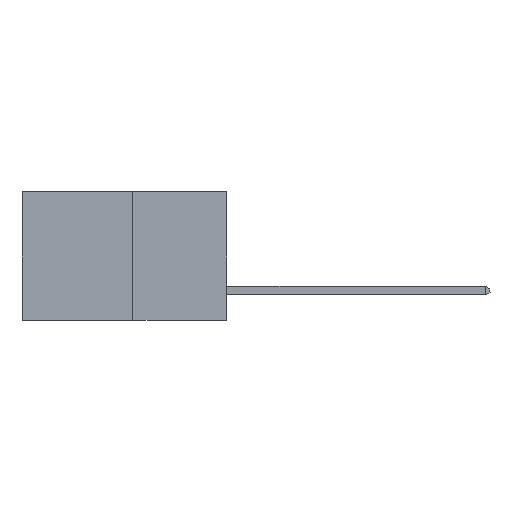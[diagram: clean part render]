
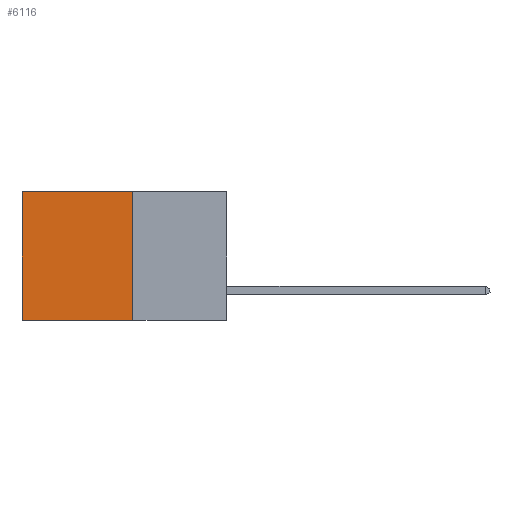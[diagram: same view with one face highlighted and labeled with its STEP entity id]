
A CAD part, left-side view. The second image highlights one B-rep face of the part: STEP entity #6116.
In plain terms, the highlighted planar face has unit normal (-1, 0, 0).
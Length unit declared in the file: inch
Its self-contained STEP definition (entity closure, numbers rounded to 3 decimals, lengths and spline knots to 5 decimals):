
#478 = LINE ( 'NONE', #4108, #4606 ) ;
#714 = ORIENTED_EDGE ( 'NONE', *, *, #7347, .T. ) ;
#821 = ORIENTED_EDGE ( 'NONE', *, *, #3410, .F. ) ;
#1174 = EDGE_CURVE ( 'NONE', #5938, #10491, #3678, .T. ) ;
#1393 = VECTOR ( 'NONE', #8315, 39.37008 ) ;
#1522 = VECTOR ( 'NONE', #7746, 39.37008 ) ;
#1723 = CARTESIAN_POINT ( 'NONE',  ( 0.277, 0.27, 0. ) ) ;
#1816 = LINE ( 'NONE', #4762, #6159 ) ;
#1988 = VERTEX_POINT ( 'NONE', #9669 ) ;
#2504 = FACE_OUTER_BOUND ( 'NONE', #3610, .T. ) ;
#2809 = ORIENTED_EDGE ( 'NONE', *, *, #1174, .F. ) ;
#3410 = EDGE_CURVE ( 'NONE', #1988, #5938, #1816, .T. ) ;
#3530 = LINE ( 'NONE', #1723, #1522 ) ;
#3610 = EDGE_LOOP ( 'NONE', ( #3947, #2809, #821, #714 ) ) ;
#3678 = LINE ( 'NONE', #8778, #1393 ) ;
#3947 = ORIENTED_EDGE ( 'NONE', *, *, #10653, .T. ) ;
#4108 = CARTESIAN_POINT ( 'NONE',  ( 0.277, 0.59, -0.37 ) ) ;
#4606 = VECTOR ( 'NONE', #10739, 39.37008 ) ;
#4744 = DIRECTION ( 'NONE',  ( 0., 0., -1. ) ) ;
#4762 = CARTESIAN_POINT ( 'NONE',  ( 0.277, 0.27, -0.37 ) ) ;
#4779 = DIRECTION ( 'NONE',  ( 0., 0., -1. ) ) ;
#4844 = DIRECTION ( 'NONE',  ( 1., 0., 0. ) ) ;
#5301 = CARTESIAN_POINT ( 'NONE',  ( 0.277, 0.27, -0.37 ) ) ;
#5938 = VERTEX_POINT ( 'NONE', #7079 ) ;
#5948 = PLANE ( 'NONE',  #10227 ) ;
#6116 = ADVANCED_FACE ( 'NONE', ( #2504 ), #5948, .F. ) ;
#6159 = VECTOR ( 'NONE', #4744, 39.37008 ) ;
#7079 = CARTESIAN_POINT ( 'NONE',  ( 0.277, 0.27, -0.37 ) ) ;
#7347 = EDGE_CURVE ( 'NONE', #1988, #7781, #3530, .T. ) ;
#7619 = CARTESIAN_POINT ( 'NONE',  ( 0.277, 0.59, -0.37 ) ) ;
#7746 = DIRECTION ( 'NONE',  ( 0., 1., 0. ) ) ;
#7781 = VERTEX_POINT ( 'NONE', #8865 ) ;
#8315 = DIRECTION ( 'NONE',  ( 0., 1., 0. ) ) ;
#8778 = CARTESIAN_POINT ( 'NONE',  ( 0.277, 0.27, -0.37 ) ) ;
#8865 = CARTESIAN_POINT ( 'NONE',  ( 0.277, 0.59, 0. ) ) ;
#9669 = CARTESIAN_POINT ( 'NONE',  ( 0.277, 0.27, 0. ) ) ;
#10227 = AXIS2_PLACEMENT_3D ( 'NONE', #5301, #4844, #4779 ) ;
#10491 = VERTEX_POINT ( 'NONE', #7619 ) ;
#10653 = EDGE_CURVE ( 'NONE', #7781, #10491, #478, .T. ) ;
#10739 = DIRECTION ( 'NONE',  ( 0., 0., -1. ) ) ;
